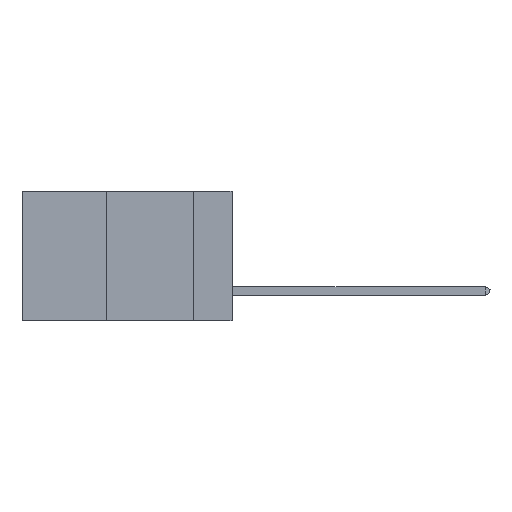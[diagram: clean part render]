
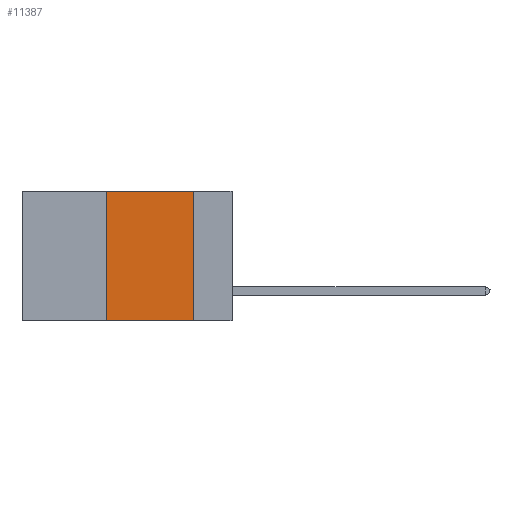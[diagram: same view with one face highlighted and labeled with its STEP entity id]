
A CAD part, left-side view. The second image highlights one B-rep face of the part: STEP entity #11387.
In plain terms, the highlighted planar face has unit normal (-1, 0, 0).
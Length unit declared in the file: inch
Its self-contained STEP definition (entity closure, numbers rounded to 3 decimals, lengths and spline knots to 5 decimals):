
#1344 = VECTOR ( 'NONE', #28486, 39.37008 ) ;
#3694 = CARTESIAN_POINT ( 'NONE',  ( 0., 0.11, -0.37 ) ) ;
#3709 = VECTOR ( 'NONE', #34743, 39.37008 ) ;
#6055 = FACE_OUTER_BOUND ( 'NONE', #21704, .T. ) ;
#7451 = CARTESIAN_POINT ( 'NONE',  ( 0., 0.11, 0. ) ) ;
#9313 = LINE ( 'NONE', #37572, #1344 ) ;
#10691 = VERTEX_POINT ( 'NONE', #36034 ) ;
#10712 = CARTESIAN_POINT ( 'NONE',  ( 0., 0.11, 0. ) ) ;
#11303 = DIRECTION ( 'NONE',  ( 0., 0., -1. ) ) ;
#11387 = ADVANCED_FACE ( 'NONE', ( #6055 ), #23496, .F. ) ;
#11666 = DIRECTION ( 'NONE',  ( 0., -1., 0. ) ) ;
#11919 = CARTESIAN_POINT ( 'NONE',  ( 0., 0.6, -0.37 ) ) ;
#11966 = LINE ( 'NONE', #11919, #29327 ) ;
#11985 = VERTEX_POINT ( 'NONE', #3694 ) ;
#12709 = AXIS2_PLACEMENT_3D ( 'NONE', #29538, #20609, #11303 ) ;
#14011 = CARTESIAN_POINT ( 'NONE',  ( 0., 0.6, 0. ) ) ;
#14396 = LINE ( 'NONE', #14011, #22851 ) ;
#15505 = EDGE_CURVE ( 'NONE', #10691, #34313, #14396, .T. ) ;
#15526 = ORIENTED_EDGE ( 'NONE', *, *, #24261, .F. ) ;
#16929 = ORIENTED_EDGE ( 'NONE', *, *, #35130, .F. ) ;
#17337 = EDGE_CURVE ( 'NONE', #19416, #11985, #11966, .T. ) ;
#19164 = ORIENTED_EDGE ( 'NONE', *, *, #15505, .F. ) ;
#19416 = VERTEX_POINT ( 'NONE', #32270 ) ;
#20609 = DIRECTION ( 'NONE',  ( 1., 0., 0. ) ) ;
#21400 = ORIENTED_EDGE ( 'NONE', *, *, #17337, .T. ) ;
#21704 = EDGE_LOOP ( 'NONE', ( #15526, #19164, #16929, #21400 ) ) ;
#22539 = DIRECTION ( 'NONE',  ( 0., -1., 0. ) ) ;
#22851 = VECTOR ( 'NONE', #22539, 39.37008 ) ;
#23496 = PLANE ( 'NONE',  #12709 ) ;
#24261 = EDGE_CURVE ( 'NONE', #34313, #11985, #26284, .T. ) ;
#26284 = LINE ( 'NONE', #10712, #3709 ) ;
#28486 = DIRECTION ( 'NONE',  ( 0., 0., 1. ) ) ;
#29327 = VECTOR ( 'NONE', #11666, 39.37008 ) ;
#29538 = CARTESIAN_POINT ( 'NONE',  ( 0., 0.6, 0. ) ) ;
#32270 = CARTESIAN_POINT ( 'NONE',  ( 0., 0.36, -0.37 ) ) ;
#34313 = VERTEX_POINT ( 'NONE', #7451 ) ;
#34743 = DIRECTION ( 'NONE',  ( 0., 0., -1. ) ) ;
#35130 = EDGE_CURVE ( 'NONE', #19416, #10691, #9313, .T. ) ;
#36034 = CARTESIAN_POINT ( 'NONE',  ( 0., 0.36, 0. ) ) ;
#37572 = CARTESIAN_POINT ( 'NONE',  ( 0., 0.36, 0. ) ) ;
